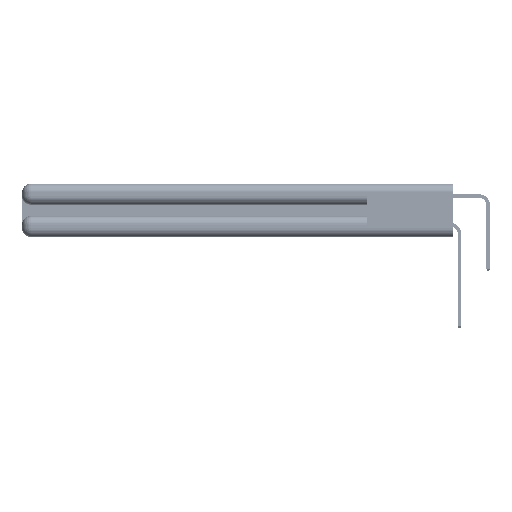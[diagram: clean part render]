
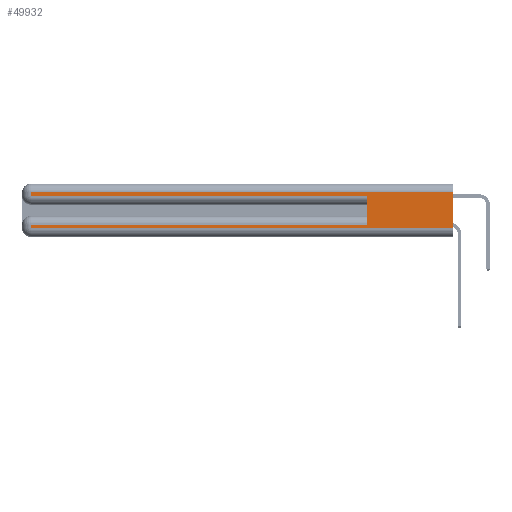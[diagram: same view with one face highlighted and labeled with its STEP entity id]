
A CAD part, left-side view. The second image highlights one B-rep face of the part: STEP entity #49932.
In plain terms, the highlighted planar face has unit normal (-1, 0, 0).
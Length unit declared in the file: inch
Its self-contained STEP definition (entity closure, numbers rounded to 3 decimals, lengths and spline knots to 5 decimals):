
#340 = VERTEX_POINT ( 'NONE', #35473 ) ;
#610 = VECTOR ( 'NONE', #32595, 39.37008 ) ;
#1040 = VERTEX_POINT ( 'NONE', #31732 ) ;
#1424 = VERTEX_POINT ( 'NONE', #2539 ) ;
#2539 = CARTESIAN_POINT ( 'NONE',  ( 0., 0., 0.31 ) ) ;
#3193 = ORIENTED_EDGE ( 'NONE', *, *, #16296, .T. ) ;
#4027 = LINE ( 'NONE', #45418, #610 ) ;
#5003 = VECTOR ( 'NONE', #55614, 39.37008 ) ;
#6647 = CARTESIAN_POINT ( 'NONE',  ( 0., 0., 0.06 ) ) ;
#6892 = DIRECTION ( 'NONE',  ( 0., -1., 0. ) ) ;
#6970 = CARTESIAN_POINT ( 'NONE',  ( 0., 0., 0.31 ) ) ;
#7041 = FACE_OUTER_BOUND ( 'NONE', #34934, .T. ) ;
#7300 = CARTESIAN_POINT ( 'NONE',  ( 0., 2.94, 0.06 ) ) ;
#7586 = VERTEX_POINT ( 'NONE', #6647 ) ;
#9002 = VECTOR ( 'NONE', #26892, 39.37008 ) ;
#12160 = DIRECTION ( 'NONE',  ( 0., 0., -1. ) ) ;
#12408 = EDGE_CURVE ( 'NONE', #340, #12833, #16504, .T. ) ;
#12443 = AXIS2_PLACEMENT_3D ( 'NONE', #35482, #14278, #44544 ) ;
#12833 = VERTEX_POINT ( 'NONE', #7300 ) ;
#13078 = VECTOR ( 'NONE', #51636, 39.37008 ) ;
#13600 = ORIENTED_EDGE ( 'NONE', *, *, #31575, .F. ) ;
#14278 = DIRECTION ( 'NONE',  ( 1., 0., 0. ) ) ;
#14969 = LINE ( 'NONE', #6970, #36008 ) ;
#15476 = DIRECTION ( 'NONE',  ( 0., 1., 0. ) ) ;
#16296 = EDGE_CURVE ( 'NONE', #20619, #46088, #31186, .T. ) ;
#16504 = LINE ( 'NONE', #51224, #5003 ) ;
#20619 = VERTEX_POINT ( 'NONE', #54154 ) ;
#21387 = CARTESIAN_POINT ( 'NONE',  ( 0., 0.6, 0.145 ) ) ;
#24258 = VECTOR ( 'NONE', #15476, 39.37008 ) ;
#24906 = EDGE_CURVE ( 'NONE', #12833, #7586, #45615, .T. ) ;
#25567 = EDGE_CURVE ( 'NONE', #1040, #44416, #54314, .T. ) ;
#26311 = ORIENTED_EDGE ( 'NONE', *, *, #27310, .T. ) ;
#26836 = ORIENTED_EDGE ( 'NONE', *, *, #24906, .T. ) ;
#26892 = DIRECTION ( 'NONE',  ( 0., 0., -1. ) ) ;
#27310 = EDGE_CURVE ( 'NONE', #1424, #20619, #14969, .T. ) ;
#28695 = VECTOR ( 'NONE', #6892, 39.37008 ) ;
#29032 = CARTESIAN_POINT ( 'NONE',  ( 0., 0., 0.06 ) ) ;
#30099 = CARTESIAN_POINT ( 'NONE',  ( 0., 0.6, 0.285 ) ) ;
#31186 = LINE ( 'NONE', #46753, #54800 ) ;
#31575 = EDGE_CURVE ( 'NONE', #1424, #7586, #51633, .T. ) ;
#31732 = CARTESIAN_POINT ( 'NONE',  ( 0., 0.6, 0.085 ) ) ;
#32595 = DIRECTION ( 'NONE',  ( 0., -1., 0. ) ) ;
#34287 = ORIENTED_EDGE ( 'NONE', *, *, #12408, .T. ) ;
#34934 = EDGE_LOOP ( 'NONE', ( #13600, #26311, #3193, #36840, #47513, #51493, #34287, #26836 ) ) ;
#35473 = CARTESIAN_POINT ( 'NONE',  ( 0., 2.94, 0.085 ) ) ;
#35482 = CARTESIAN_POINT ( 'NONE',  ( 0., 0., 0.37 ) ) ;
#36008 = VECTOR ( 'NONE', #42147, 39.37008 ) ;
#36071 = EDGE_CURVE ( 'NONE', #46088, #44416, #4027, .T. ) ;
#36840 = ORIENTED_EDGE ( 'NONE', *, *, #36071, .T. ) ;
#39361 = CARTESIAN_POINT ( 'NONE',  ( 0., 2.94, 0.285 ) ) ;
#40190 = PLANE ( 'NONE',  #12443 ) ;
#41405 = CARTESIAN_POINT ( 'NONE',  ( 0., 0., 0.085 ) ) ;
#42147 = DIRECTION ( 'NONE',  ( 0., 1., 0. ) ) ;
#44416 = VERTEX_POINT ( 'NONE', #30099 ) ;
#44544 = DIRECTION ( 'NONE',  ( 0., 0., -1. ) ) ;
#45418 = CARTESIAN_POINT ( 'NONE',  ( 0., 0., 0.285 ) ) ;
#45615 = LINE ( 'NONE', #29032, #28695 ) ;
#46088 = VERTEX_POINT ( 'NONE', #39361 ) ;
#46355 = EDGE_CURVE ( 'NONE', #1040, #340, #51329, .T. ) ;
#46753 = CARTESIAN_POINT ( 'NONE',  ( 0., 2.94, 0.37 ) ) ;
#47513 = ORIENTED_EDGE ( 'NONE', *, *, #25567, .F. ) ;
#49932 = ADVANCED_FACE ( 'NONE', ( #7041 ), #40190, .F. ) ;
#51224 = CARTESIAN_POINT ( 'NONE',  ( 0., 2.94, 0.37 ) ) ;
#51329 = LINE ( 'NONE', #41405, #24258 ) ;
#51493 = ORIENTED_EDGE ( 'NONE', *, *, #46355, .T. ) ;
#51633 = LINE ( 'NONE', #52432, #9002 ) ;
#51636 = DIRECTION ( 'NONE',  ( 0., 0., 1. ) ) ;
#52432 = CARTESIAN_POINT ( 'NONE',  ( 0., 0., 0.37 ) ) ;
#54154 = CARTESIAN_POINT ( 'NONE',  ( 0., 2.94, 0.31 ) ) ;
#54314 = LINE ( 'NONE', #21387, #13078 ) ;
#54800 = VECTOR ( 'NONE', #12160, 39.37008 ) ;
#55614 = DIRECTION ( 'NONE',  ( 0., 0., -1. ) ) ;
